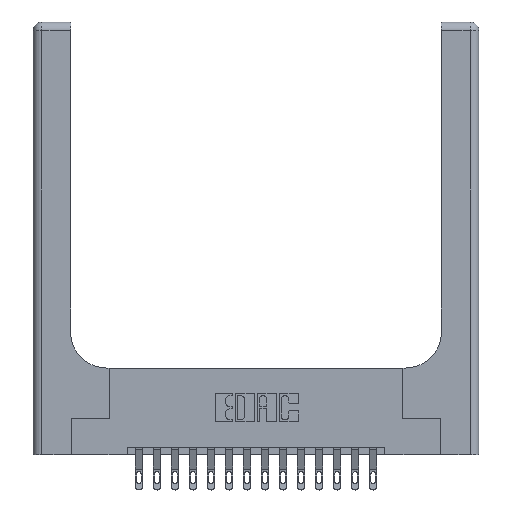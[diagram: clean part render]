
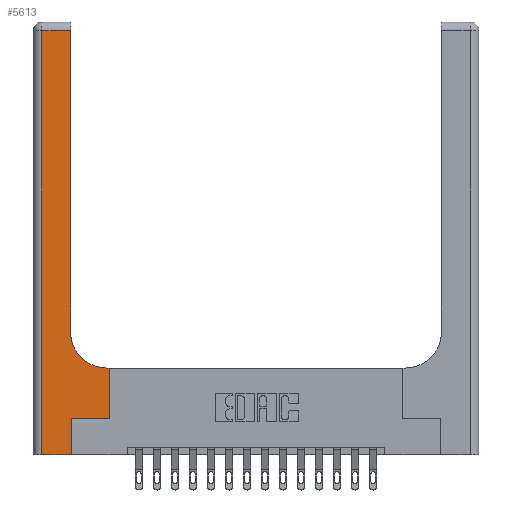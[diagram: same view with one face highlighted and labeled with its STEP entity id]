
A CAD part, top view. The second image highlights one B-rep face of the part: STEP entity #5613.
In plain terms, the highlighted planar face has unit normal (0, 0, 1).
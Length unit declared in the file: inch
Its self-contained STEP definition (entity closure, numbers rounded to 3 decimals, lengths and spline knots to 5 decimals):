
#10 = DIRECTION ( 'NONE',  ( 1., 0., 0. ) ) ;
#47 = ORIENTED_EDGE ( 'NONE', *, *, #7467, .T. ) ;
#488 = FACE_OUTER_BOUND ( 'NONE', #13188, .T. ) ;
#760 = EDGE_CURVE ( 'NONE', #18288, #17035, #9351, .T. ) ;
#903 = CARTESIAN_POINT ( 'NONE',  ( 0., 2.94, 0.37 ) ) ;
#1299 = VECTOR ( 'NONE', #8551, 39.37008 ) ;
#1357 = VERTEX_POINT ( 'NONE', #2165 ) ;
#1515 = ORIENTED_EDGE ( 'NONE', *, *, #12065, .T. ) ;
#1566 = CARTESIAN_POINT ( 'NONE',  ( 0.265, 0., 0.37 ) ) ;
#2018 = PLANE ( 'NONE',  #3999 ) ;
#2081 = ORIENTED_EDGE ( 'NONE', *, *, #17946, .T. ) ;
#2163 = LINE ( 'NONE', #903, #8620 ) ;
#2165 = CARTESIAN_POINT ( 'NONE',  ( 0.26, 2.94, 0.37 ) ) ;
#2221 = VERTEX_POINT ( 'NONE', #17001 ) ;
#2283 = CARTESIAN_POINT ( 'NONE',  ( 0.26, 3., 0.37 ) ) ;
#2372 = ORIENTED_EDGE ( 'NONE', *, *, #760, .T. ) ;
#2868 = CARTESIAN_POINT ( 'NONE',  ( 0.265, 0.25, 0.37 ) ) ;
#3088 = EDGE_CURVE ( 'NONE', #17035, #11331, #3165, .T. ) ;
#3165 = LINE ( 'NONE', #9048, #10115 ) ;
#3231 = CARTESIAN_POINT ( 'NONE',  ( 0.265, 0.25, 0.37 ) ) ;
#3293 = CARTESIAN_POINT ( 'NONE',  ( 0.528, 0.6, 0.37 ) ) ;
#3762 = VERTEX_POINT ( 'NONE', #15706 ) ;
#3999 = AXIS2_PLACEMENT_3D ( 'NONE', #6448, #13773, #11012 ) ;
#4727 = ORIENTED_EDGE ( 'NONE', *, *, #3088, .T. ) ;
#4882 = VECTOR ( 'NONE', #15988, 39.37008 ) ;
#5016 = VERTEX_POINT ( 'NONE', #3293 ) ;
#5383 = DIRECTION ( 'NONE',  ( 0., 1., 0. ) ) ;
#5483 = EDGE_CURVE ( 'NONE', #1357, #14019, #2163, .T. ) ;
#5613 = ADVANCED_FACE ( 'NONE', ( #488 ), #2018, .F. ) ;
#5670 = VECTOR ( 'NONE', #6712, 39.37008 ) ;
#5671 = CARTESIAN_POINT ( 'NONE',  ( 0.06, 3., 0.37 ) ) ;
#5875 = CARTESIAN_POINT ( 'NONE',  ( 0.06, 2.94, 0.37 ) ) ;
#6448 = CARTESIAN_POINT ( 'NONE',  ( 0., 3., 0.37 ) ) ;
#6511 = VECTOR ( 'NONE', #5383, 39.37008 ) ;
#6633 = LINE ( 'NONE', #16917, #6511 ) ;
#6712 = DIRECTION ( 'NONE',  ( 0., 1., 0. ) ) ;
#7467 = EDGE_CURVE ( 'NONE', #2221, #5016, #6633, .T. ) ;
#7666 = EDGE_CURVE ( 'NONE', #11331, #2221, #18721, .T. ) ;
#7687 = CARTESIAN_POINT ( 'NONE',  ( 0.26, 0.6, 0.37 ) ) ;
#8165 = LINE ( 'NONE', #2283, #5670 ) ;
#8551 = DIRECTION ( 'NONE',  ( 1., 0., 0. ) ) ;
#8620 = VECTOR ( 'NONE', #15367, 39.37008 ) ;
#9048 = CARTESIAN_POINT ( 'NONE',  ( 0.265, 0., 0.37 ) ) ;
#9351 = LINE ( 'NONE', #18071, #15353 ) ;
#10115 = VECTOR ( 'NONE', #13512, 39.37008 ) ;
#10270 = CIRCLE ( 'NONE', #17526, 0.25 ) ;
#10646 = ORIENTED_EDGE ( 'NONE', *, *, #7666, .T. ) ;
#10693 = EDGE_CURVE ( 'NONE', #14159, #1357, #8165, .T. ) ;
#10716 = VECTOR ( 'NONE', #12331, 39.37008 ) ;
#11012 = DIRECTION ( 'NONE',  ( -1., 0., 0. ) ) ;
#11331 = VERTEX_POINT ( 'NONE', #3231 ) ;
#11773 = DIRECTION ( 'NONE',  ( 0., 0., -1. ) ) ;
#11785 = CARTESIAN_POINT ( 'NONE',  ( 0.06, 0., 0.37 ) ) ;
#11874 = LINE ( 'NONE', #7687, #10716 ) ;
#12065 = EDGE_CURVE ( 'NONE', #3762, #14159, #10270, .T. ) ;
#12124 = ORIENTED_EDGE ( 'NONE', *, *, #5483, .T. ) ;
#12331 = DIRECTION ( 'NONE',  ( -1., 0., 0. ) ) ;
#12951 = CARTESIAN_POINT ( 'NONE',  ( 0.26, 0.85, 0.37 ) ) ;
#13188 = EDGE_LOOP ( 'NONE', ( #16225, #12124, #2081, #2372, #4727, #10646, #47, #18434, #1515 ) ) ;
#13512 = DIRECTION ( 'NONE',  ( 0., 1., 0. ) ) ;
#13773 = DIRECTION ( 'NONE',  ( 0., 0., -1. ) ) ;
#14019 = VERTEX_POINT ( 'NONE', #5875 ) ;
#14159 = VERTEX_POINT ( 'NONE', #12951 ) ;
#14936 = DIRECTION ( 'NONE',  ( 1., 0., 0. ) ) ;
#15353 = VECTOR ( 'NONE', #14936, 39.37008 ) ;
#15367 = DIRECTION ( 'NONE',  ( -1., 0., 0. ) ) ;
#15706 = CARTESIAN_POINT ( 'NONE',  ( 0.51, 0.6, 0.37 ) ) ;
#15988 = DIRECTION ( 'NONE',  ( 0., -1., 0. ) ) ;
#16131 = CARTESIAN_POINT ( 'NONE',  ( 0.51, 0.85, 0.37 ) ) ;
#16225 = ORIENTED_EDGE ( 'NONE', *, *, #10693, .T. ) ;
#16917 = CARTESIAN_POINT ( 'NONE',  ( 0.528, 0.25, 0.37 ) ) ;
#17001 = CARTESIAN_POINT ( 'NONE',  ( 0.528, 0.25, 0.37 ) ) ;
#17035 = VERTEX_POINT ( 'NONE', #1566 ) ;
#17288 = EDGE_CURVE ( 'NONE', #5016, #3762, #11874, .T. ) ;
#17526 = AXIS2_PLACEMENT_3D ( 'NONE', #16131, #11773, #10 ) ;
#17667 = LINE ( 'NONE', #5671, #4882 ) ;
#17946 = EDGE_CURVE ( 'NONE', #14019, #18288, #17667, .T. ) ;
#18071 = CARTESIAN_POINT ( 'NONE',  ( 0., 0., 0.37 ) ) ;
#18288 = VERTEX_POINT ( 'NONE', #11785 ) ;
#18434 = ORIENTED_EDGE ( 'NONE', *, *, #17288, .T. ) ;
#18721 = LINE ( 'NONE', #2868, #1299 ) ;
